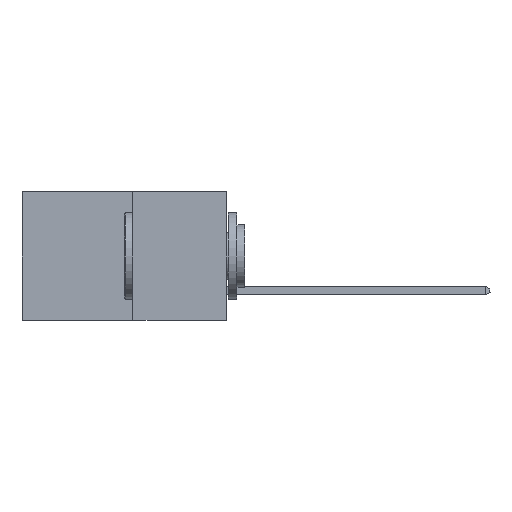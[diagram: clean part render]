
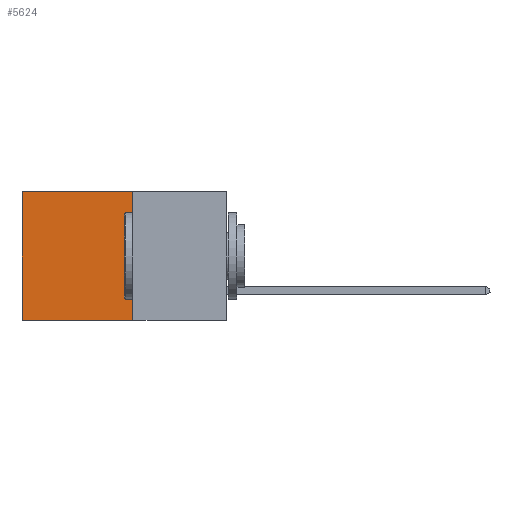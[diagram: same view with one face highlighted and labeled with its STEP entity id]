
A CAD part, left-side view. The second image highlights one B-rep face of the part: STEP entity #5624.
In plain terms, the highlighted planar face has unit normal (-1, 0, 0).
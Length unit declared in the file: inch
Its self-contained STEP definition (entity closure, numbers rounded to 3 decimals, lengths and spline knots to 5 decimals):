
#466 = DIRECTION ( 'NONE',  ( 0., 1., 0. ) ) ;
#543 = CARTESIAN_POINT ( 'NONE',  ( 0.277, 0.27, -0.37 ) ) ;
#767 = DIRECTION ( 'NONE',  ( 0., 0., -1. ) ) ;
#797 = CARTESIAN_POINT ( 'NONE',  ( 0.277, 0.59, -0.37 ) ) ;
#1560 = VERTEX_POINT ( 'NONE', #6403 ) ;
#1678 = VERTEX_POINT ( 'NONE', #24393 ) ;
#1890 = ORIENTED_EDGE ( 'NONE', *, *, #5965, .F. ) ;
#4388 = EDGE_LOOP ( 'NONE', ( #17164, #31060, #1890, #30592 ) ) ;
#5165 = CARTESIAN_POINT ( 'NONE',  ( 0.277, 0.27, 0. ) ) ;
#5624 = ADVANCED_FACE ( 'NONE', ( #11151 ), #20712, .F. ) ;
#5965 = EDGE_CURVE ( 'NONE', #18502, #20652, #26678, .T. ) ;
#6403 = CARTESIAN_POINT ( 'NONE',  ( 0.277, 0.59, 0. ) ) ;
#7021 = EDGE_CURVE ( 'NONE', #1560, #1678, #14190, .T. ) ;
#7055 = EDGE_CURVE ( 'NONE', #20652, #1678, #25862, .T. ) ;
#7759 = AXIS2_PLACEMENT_3D ( 'NONE', #20686, #20646, #20578 ) ;
#10604 = LINE ( 'NONE', #28242, #23029 ) ;
#10857 = DIRECTION ( 'NONE',  ( 0., 1., 0. ) ) ;
#10979 = CARTESIAN_POINT ( 'NONE',  ( 0.277, 0.27, -0.37 ) ) ;
#11151 = FACE_OUTER_BOUND ( 'NONE', #4388, .T. ) ;
#13419 = VECTOR ( 'NONE', #767, 39.37008 ) ;
#14190 = LINE ( 'NONE', #797, #13419 ) ;
#15688 = DIRECTION ( 'NONE',  ( 0., 0., -1. ) ) ;
#15702 = EDGE_CURVE ( 'NONE', #18502, #1560, #10604, .T. ) ;
#15803 = CARTESIAN_POINT ( 'NONE',  ( 0.277, 0.27, -0.37 ) ) ;
#17164 = ORIENTED_EDGE ( 'NONE', *, *, #7021, .T. ) ;
#18476 = VECTOR ( 'NONE', #15688, 39.37008 ) ;
#18502 = VERTEX_POINT ( 'NONE', #5165 ) ;
#20578 = DIRECTION ( 'NONE',  ( 0., 0., -1. ) ) ;
#20646 = DIRECTION ( 'NONE',  ( 1., 0., 0. ) ) ;
#20652 = VERTEX_POINT ( 'NONE', #10979 ) ;
#20686 = CARTESIAN_POINT ( 'NONE',  ( 0.277, 0.27, -0.37 ) ) ;
#20712 = PLANE ( 'NONE',  #7759 ) ;
#23029 = VECTOR ( 'NONE', #10857, 39.37008 ) ;
#24393 = CARTESIAN_POINT ( 'NONE',  ( 0.277, 0.59, -0.37 ) ) ;
#25862 = LINE ( 'NONE', #543, #31676 ) ;
#26678 = LINE ( 'NONE', #15803, #18476 ) ;
#28242 = CARTESIAN_POINT ( 'NONE',  ( 0.277, 0.27, 0. ) ) ;
#30592 = ORIENTED_EDGE ( 'NONE', *, *, #15702, .T. ) ;
#31060 = ORIENTED_EDGE ( 'NONE', *, *, #7055, .F. ) ;
#31676 = VECTOR ( 'NONE', #466, 39.37008 ) ;
